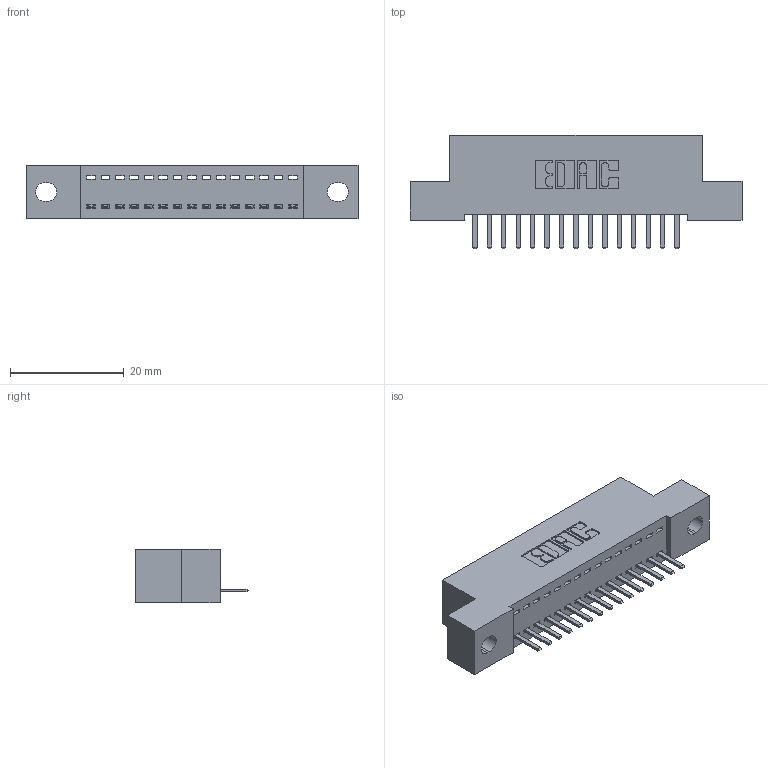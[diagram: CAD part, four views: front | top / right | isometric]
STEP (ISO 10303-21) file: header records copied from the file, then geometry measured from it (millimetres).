
FILE_DESCRIPTION (( 'STEP AP203' ), '1' );
FILE_NAME ('392-015-520-102.STEP', '2019-10-07T02:38:36', ( '' ), ( '' ), 'SwSTEP 2.0', 'SolidWorks 2016', '' );
FILE_SCHEMA (( 'CONFIG_CONTROL_DESIGN' ));
Length unit declared in the file: inch
Products named in the file (3): 392-015-520-102; 342 Part_.128 Slot; 345-292-001_345-293-120
Assembly tree (16 placements, depth 2):
  392-015-520-102
    342 Part_.128 Slot
    345-292-001_345-293-120  x15
Bounding box: 58.42 x 20.02 x 9.4 mm (x, y, z)
Volume: 4927.5 mm3; surface area: 6353.3 mm2
Topology: 16 solids, 16 shells, 1044 faces, 3071 edges, 2006 vertices
Faces by surface type: plane 730, cylinder 314
Entity records: 12779 total; most frequent: CARTESIAN_POINT 2227, ORIENTED_EDGE 2166, DIRECTION 1921, EDGE_CURVE 1083, LINE 951, VECTOR 951, VERTEX_POINT 718, AXIS2_PLACEMENT_3D 485
